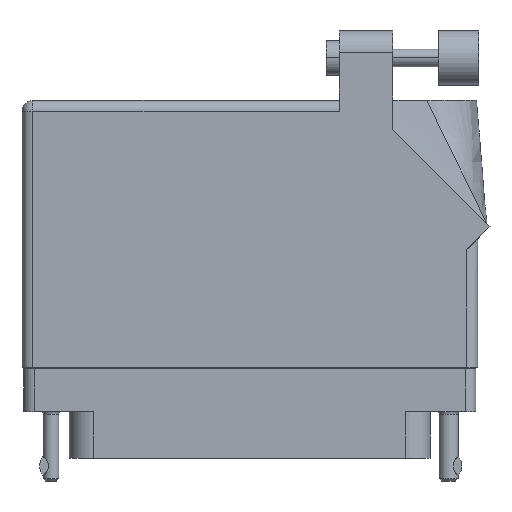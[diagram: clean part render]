
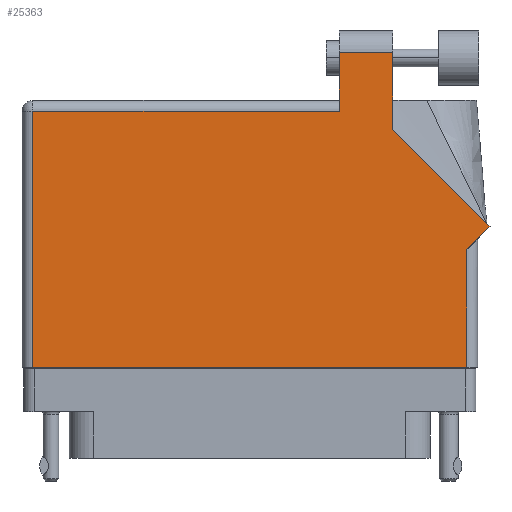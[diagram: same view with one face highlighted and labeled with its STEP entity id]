
A CAD part, front view. The second image highlights one B-rep face of the part: STEP entity #25363.
In plain terms, the highlighted face is planar.
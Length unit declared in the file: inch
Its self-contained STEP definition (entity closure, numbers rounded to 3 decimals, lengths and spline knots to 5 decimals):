
#81 = VECTOR ( 'NONE', #45468, 39.37008 ) ;
#546 = DIRECTION ( 'NONE',  ( 0., -1., 0. ) ) ;
#609 = VECTOR ( 'NONE', #38834, 39.37008 ) ;
#999 = LINE ( 'NONE', #52802, #37291 ) ;
#1072 = EDGE_CURVE ( 'NONE', #37848, #3214, #8915, .T. ) ;
#1326 = CARTESIAN_POINT ( 'NONE',  ( -1.306, -0.1, 0.455 ) ) ;
#1496 = VERTEX_POINT ( 'NONE', #53283 ) ;
#1667 = ORIENTED_EDGE ( 'NONE', *, *, #1072, .T. ) ;
#1858 = CARTESIAN_POINT ( 'NONE',  ( -1.306, 1.43, 0.455 ) ) ;
#2268 = CARTESIAN_POINT ( 'NONE',  ( 0.513, 1.43, 0.455 ) ) ;
#3214 = VERTEX_POINT ( 'NONE', #37415 ) ;
#4005 = DIRECTION ( 'NONE',  ( -0.707, 0.707, 0. ) ) ;
#5906 = PLANE ( 'NONE',  #51381 ) ;
#6250 = LINE ( 'NONE', #1326, #24716 ) ;
#6799 = CARTESIAN_POINT ( 'NONE',  ( 0.513, 1.368, 0.455 ) ) ;
#7969 = ORIENTED_EDGE ( 'NONE', *, *, #42286, .T. ) ;
#8915 = LINE ( 'NONE', #34017, #17146 ) ;
#9801 = CARTESIAN_POINT ( 'NONE',  ( -1.244, 1.368, 0.455 ) ) ;
#10895 = ORIENTED_EDGE ( 'NONE', *, *, #53424, .T. ) ;
#11967 = LINE ( 'NONE', #56378, #19414 ) ;
#12289 = CARTESIAN_POINT ( 'NONE',  ( 1.37671, 0.70771, 0.455 ) ) ;
#13020 = CARTESIAN_POINT ( 'NONE',  ( 0.513, 1.705, 0.455 ) ) ;
#13123 = LINE ( 'NONE', #2268, #81 ) ;
#13393 = VERTEX_POINT ( 'NONE', #6799 ) ;
#15659 = LINE ( 'NONE', #25065, #609 ) ;
#17146 = VECTOR ( 'NONE', #4005, 39.37008 ) ;
#17549 = CARTESIAN_POINT ( 'NONE',  ( 0.513, 1.705, 0.455 ) ) ;
#17627 = VERTEX_POINT ( 'NONE', #9801 ) ;
#18963 = CARTESIAN_POINT ( 'NONE',  ( 0.82, 1.705, 0.455 ) ) ;
#19028 = LINE ( 'NONE', #13020, #42374 ) ;
#19414 = VECTOR ( 'NONE', #47466, 39.37008 ) ;
#20974 = EDGE_CURVE ( 'NONE', #17627, #37730, #49777, .T. ) ;
#24716 = VECTOR ( 'NONE', #31739, 39.37008 ) ;
#25065 = CARTESIAN_POINT ( 'NONE',  ( -1.306, 1.368, 0.455 ) ) ;
#25363 = ADVANCED_FACE ( 'NONE', ( #34255 ), #5906, .F. ) ;
#25850 = VERTEX_POINT ( 'NONE', #18963 ) ;
#26531 = VECTOR ( 'NONE', #31045, 39.37008 ) ;
#26616 = VERTEX_POINT ( 'NONE', #17549 ) ;
#27379 = ORIENTED_EDGE ( 'NONE', *, *, #48678, .T. ) ;
#27864 = VECTOR ( 'NONE', #546, 39.37008 ) ;
#30752 = DIRECTION ( 'NONE',  ( -1., 0., 0. ) ) ;
#31045 = DIRECTION ( 'NONE',  ( 0., 1., 0. ) ) ;
#31739 = DIRECTION ( 'NONE',  ( 1., 0., 0. ) ) ;
#32786 = EDGE_CURVE ( 'NONE', #25850, #26616, #19028, .T. ) ;
#32842 = DIRECTION ( 'NONE',  ( -1., 0., 0. ) ) ;
#33050 = ORIENTED_EDGE ( 'NONE', *, *, #32786, .T. ) ;
#34017 = CARTESIAN_POINT ( 'NONE',  ( 1.37671, 0.70771, 0.455 ) ) ;
#34255 = FACE_OUTER_BOUND ( 'NONE', #55368, .T. ) ;
#36462 = DIRECTION ( 'NONE',  ( 0., 0., -1. ) ) ;
#37291 = VECTOR ( 'NONE', #48637, 39.37008 ) ;
#37415 = CARTESIAN_POINT ( 'NONE',  ( 0.82, 1.26442, 0.455 ) ) ;
#37730 = VERTEX_POINT ( 'NONE', #55434 ) ;
#37848 = VERTEX_POINT ( 'NONE', #12289 ) ;
#37869 = ORIENTED_EDGE ( 'NONE', *, *, #56438, .T. ) ;
#38834 = DIRECTION ( 'NONE',  ( -1., 0., 0. ) ) ;
#40176 = ORIENTED_EDGE ( 'NONE', *, *, #43120, .T. ) ;
#40419 = ORIENTED_EDGE ( 'NONE', *, *, #52852, .T. ) ;
#41039 = ORIENTED_EDGE ( 'NONE', *, *, #20974, .T. ) ;
#42286 = EDGE_CURVE ( 'NONE', #3214, #25850, #42982, .T. ) ;
#42374 = VECTOR ( 'NONE', #30752, 39.37008 ) ;
#42982 = LINE ( 'NONE', #44296, #26531 ) ;
#43120 = EDGE_CURVE ( 'NONE', #13393, #17627, #15659, .T. ) ;
#44296 = CARTESIAN_POINT ( 'NONE',  ( 0.82, 1.26442, 0.455 ) ) ;
#45468 = DIRECTION ( 'NONE',  ( 0., -1., 0. ) ) ;
#47281 = VERTEX_POINT ( 'NONE', #56306 ) ;
#47466 = DIRECTION ( 'NONE',  ( 0., 1., 0. ) ) ;
#48637 = DIRECTION ( 'NONE',  ( 0.707, 0.707, 0. ) ) ;
#48678 = EDGE_CURVE ( 'NONE', #26616, #13393, #13123, .T. ) ;
#49777 = LINE ( 'NONE', #53115, #27864 ) ;
#51381 = AXIS2_PLACEMENT_3D ( 'NONE', #1858, #36462, #32842 ) ;
#52802 = CARTESIAN_POINT ( 'NONE',  ( 1.306, 0.637, 0.455 ) ) ;
#52852 = EDGE_CURVE ( 'NONE', #1496, #37848, #999, .T. ) ;
#53115 = CARTESIAN_POINT ( 'NONE',  ( -1.244, -0.1, 0.455 ) ) ;
#53283 = CARTESIAN_POINT ( 'NONE',  ( 1.244, 0.575, 0.455 ) ) ;
#53424 = EDGE_CURVE ( 'NONE', #47281, #1496, #11967, .T. ) ;
#55368 = EDGE_LOOP ( 'NONE', ( #7969, #33050, #27379, #40176, #41039, #37869, #10895, #40419, #1667 ) ) ;
#55434 = CARTESIAN_POINT ( 'NONE',  ( -1.244, -0.1, 0.455 ) ) ;
#56306 = CARTESIAN_POINT ( 'NONE',  ( 1.244, -0.1, 0.455 ) ) ;
#56378 = CARTESIAN_POINT ( 'NONE',  ( 1.244, 0.637, 0.455 ) ) ;
#56438 = EDGE_CURVE ( 'NONE', #37730, #47281, #6250, .T. ) ;
